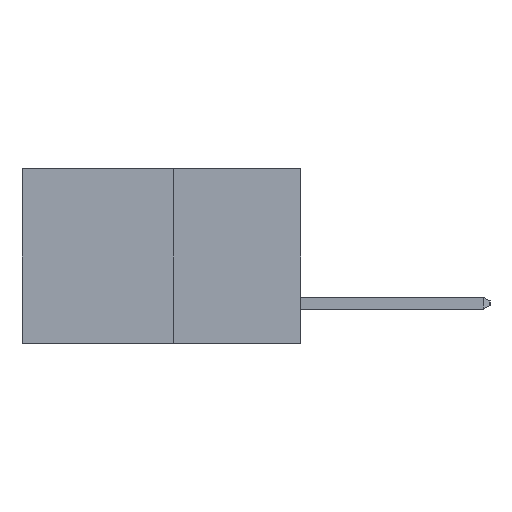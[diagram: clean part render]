
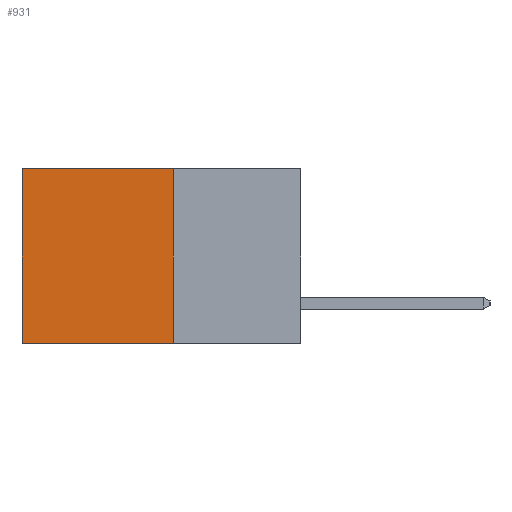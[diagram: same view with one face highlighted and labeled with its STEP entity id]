
A CAD part, left-side view. The second image highlights one B-rep face of the part: STEP entity #931.
In plain terms, the highlighted planar face has unit normal (-1, 0, 0).
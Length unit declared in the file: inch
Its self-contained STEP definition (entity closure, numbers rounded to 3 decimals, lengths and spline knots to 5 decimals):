
#254 = VERTEX_POINT ( 'NONE', #11162 ) ;
#756 = LINE ( 'NONE', #12114, #12149 ) ;
#931 = ADVANCED_FACE ( 'NONE', ( #3604 ), #11400, .F. ) ;
#1062 = DIRECTION ( 'NONE',  ( 0., 1., 0. ) ) ;
#1575 = CARTESIAN_POINT ( 'NONE',  ( 0.277, 0.59, -0.37 ) ) ;
#1686 = VECTOR ( 'NONE', #6047, 39.37008 ) ;
#3604 = FACE_OUTER_BOUND ( 'NONE', #7812, .T. ) ;
#4143 = EDGE_CURVE ( 'NONE', #6645, #6333, #13030, .T. ) ;
#4825 = LINE ( 'NONE', #8258, #12531 ) ;
#5071 = VERTEX_POINT ( 'NONE', #10172 ) ;
#5085 = CARTESIAN_POINT ( 'NONE',  ( 0.277, 0.27, 0. ) ) ;
#6047 = DIRECTION ( 'NONE',  ( 0., 0., -1. ) ) ;
#6173 = CARTESIAN_POINT ( 'NONE',  ( 0.277, 0.27, -0.37 ) ) ;
#6263 = LINE ( 'NONE', #1575, #9582 ) ;
#6333 = VERTEX_POINT ( 'NONE', #12224 ) ;
#6645 = VERTEX_POINT ( 'NONE', #5085 ) ;
#7228 = ORIENTED_EDGE ( 'NONE', *, *, #4143, .F. ) ;
#7812 = EDGE_LOOP ( 'NONE', ( #9884, #11714, #7228, #12593 ) ) ;
#8258 = CARTESIAN_POINT ( 'NONE',  ( 0.277, 0.27, 0. ) ) ;
#8460 = EDGE_CURVE ( 'NONE', #254, #5071, #6263, .T. ) ;
#9376 = DIRECTION ( 'NONE',  ( 0., 0., -1. ) ) ;
#9582 = VECTOR ( 'NONE', #9376, 39.37008 ) ;
#9884 = ORIENTED_EDGE ( 'NONE', *, *, #8460, .T. ) ;
#10172 = CARTESIAN_POINT ( 'NONE',  ( 0.277, 0.59, -0.37 ) ) ;
#10273 = EDGE_CURVE ( 'NONE', #6645, #254, #4825, .T. ) ;
#10458 = DIRECTION ( 'NONE',  ( 0., 1., 0. ) ) ;
#11162 = CARTESIAN_POINT ( 'NONE',  ( 0.277, 0.59, 0. ) ) ;
#11400 = PLANE ( 'NONE',  #11463 ) ;
#11463 = AXIS2_PLACEMENT_3D ( 'NONE', #11592, #13332, #13036 ) ;
#11592 = CARTESIAN_POINT ( 'NONE',  ( 0.277, 0.27, -0.37 ) ) ;
#11714 = ORIENTED_EDGE ( 'NONE', *, *, #12229, .F. ) ;
#12114 = CARTESIAN_POINT ( 'NONE',  ( 0.277, 0.27, -0.37 ) ) ;
#12149 = VECTOR ( 'NONE', #1062, 39.37008 ) ;
#12224 = CARTESIAN_POINT ( 'NONE',  ( 0.277, 0.27, -0.37 ) ) ;
#12229 = EDGE_CURVE ( 'NONE', #6333, #5071, #756, .T. ) ;
#12531 = VECTOR ( 'NONE', #10458, 39.37008 ) ;
#12593 = ORIENTED_EDGE ( 'NONE', *, *, #10273, .T. ) ;
#13030 = LINE ( 'NONE', #6173, #1686 ) ;
#13036 = DIRECTION ( 'NONE',  ( 0., 0., -1. ) ) ;
#13332 = DIRECTION ( 'NONE',  ( 1., 0., 0. ) ) ;
